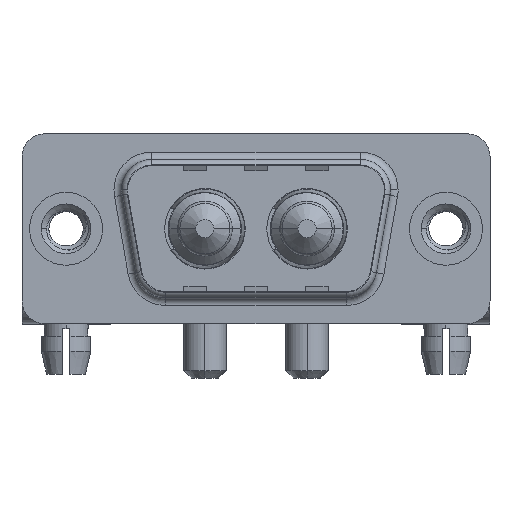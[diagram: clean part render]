
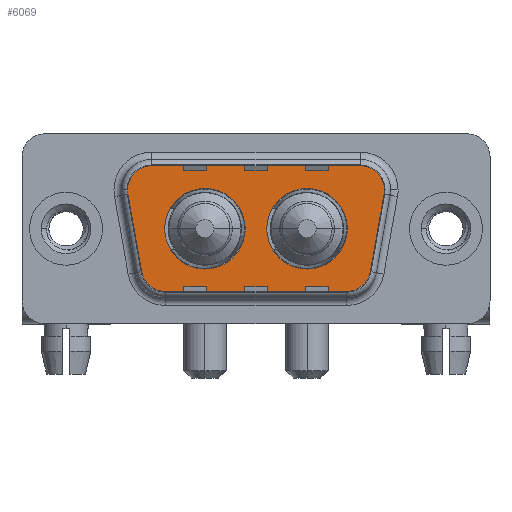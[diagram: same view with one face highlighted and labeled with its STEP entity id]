
A CAD part, top view. The second image highlights one B-rep face of the part: STEP entity #6069.
In plain terms, the highlighted planar face has unit normal (0, 0, 1).
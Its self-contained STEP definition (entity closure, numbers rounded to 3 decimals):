
#270 = CIRCLE ( 'NONE', #10573, 2.65 ) ;
#485 = EDGE_CURVE ( 'NONE', #7321, #1533, #10133, .T. ) ;
#547 = CARTESIAN_POINT ( 'NONE',  ( 9.14, 0., 0. ) ) ;
#634 = VERTEX_POINT ( 'NONE', #9031 ) ;
#652 = AXIS2_PLACEMENT_3D ( 'NONE', #2389, #12251, #5765 ) ;
#685 = CIRCLE ( 'NONE', #13938, 2.65 ) ;
#824 = LINE ( 'NONE', #10684, #3923 ) ;
#887 = DIRECTION ( 'NONE',  ( 0.174, 0.985, 0. ) ) ;
#907 = DIRECTION ( 'NONE',  ( 1., 0., 0. ) ) ;
#1117 = ORIENTED_EDGE ( 'NONE', *, *, #485, .T. ) ;
#1237 = EDGE_CURVE ( 'NONE', #4192, #14026, #5789, .T. ) ;
#1302 = ORIENTED_EDGE ( 'NONE', *, *, #2792, .T. ) ;
#1533 = VERTEX_POINT ( 'NONE', #12613 ) ;
#1662 = ORIENTED_EDGE ( 'NONE', *, *, #10851, .T. ) ;
#1864 = CARTESIAN_POINT ( 'NONE',  ( 18.51, 0., 0. ) ) ;
#2074 = CARTESIAN_POINT ( 'NONE',  ( 9.14, 0., 0. ) ) ;
#2175 = DIRECTION ( 'NONE',  ( -1., 0., 0. ) ) ;
#2204 = DIRECTION ( 'NONE',  ( -1., 0., 0. ) ) ;
#2281 = AXIS2_PLACEMENT_3D ( 'NONE', #3483, #10144, #3620 ) ;
#2372 = DIRECTION ( 'NONE',  ( 0., 0., 1. ) ) ;
#2389 = CARTESIAN_POINT ( 'NONE',  ( 18.541, -2.9, 0. ) ) ;
#2602 = DIRECTION ( 'NONE',  ( 0., 0., 1. ) ) ;
#2766 = CIRCLE ( 'NONE', #13952, 2. ) ;
#2767 = DIRECTION ( 'NONE',  ( 0., 0., 1. ) ) ;
#2792 = EDGE_CURVE ( 'NONE', #11242, #5086, #8557, .T. ) ;
#3089 = EDGE_CURVE ( 'NONE', #634, #4227, #270, .T. ) ;
#3205 = EDGE_LOOP ( 'NONE', ( #7074, #8288 ) ) ;
#3242 = CARTESIAN_POINT ( 'NONE',  ( 19.564, 2.9, 0. ) ) ;
#3483 = CARTESIAN_POINT ( 'NONE',  ( 6.459, -2.9, 0. ) ) ;
#3620 = DIRECTION ( 'NONE',  ( -1., 0., 0. ) ) ;
#3659 = EDGE_CURVE ( 'NONE', #4227, #634, #685, .T. ) ;
#3923 = VECTOR ( 'NONE', #887, 1000. ) ;
#3963 = DIRECTION ( 'NONE',  ( 1., 0., 0. ) ) ;
#4192 = VERTEX_POINT ( 'NONE', #13321 ) ;
#4227 = VERTEX_POINT ( 'NONE', #7830 ) ;
#4237 = EDGE_CURVE ( 'NONE', #5086, #11432, #10915, .T. ) ;
#4302 = CARTESIAN_POINT ( 'NONE',  ( 3.466, 2.553, 0. ) ) ;
#4354 = CIRCLE ( 'NONE', #10530, 2.65 ) ;
#4402 = VERTEX_POINT ( 'NONE', #4816 ) ;
#4488 = LINE ( 'NONE', #11137, #9179 ) ;
#4498 = CARTESIAN_POINT ( 'NONE',  ( 18.541, -4.9, 0. ) ) ;
#4816 = CARTESIAN_POINT ( 'NONE',  ( 21.534, 2.553, 0. ) ) ;
#5084 = AXIS2_PLACEMENT_3D ( 'NONE', #7219, #2767, #7148 ) ;
#5086 = VERTEX_POINT ( 'NONE', #4498 ) ;
#5178 = EDGE_LOOP ( 'NONE', ( #13617, #1662, #7521, #1117, #10846, #5737, #11126, #7976, #1302 ) ) ;
#5289 = VERTEX_POINT ( 'NONE', #11369 ) ;
#5326 = CARTESIAN_POINT ( 'NONE',  ( 19.564, 2.9, 0. ) ) ;
#5380 = VECTOR ( 'NONE', #13698, 1000. ) ;
#5528 = CARTESIAN_POINT ( 'NONE',  ( 21.564, 2.9, 0. ) ) ;
#5575 = DIRECTION ( 'NONE',  ( 0., 0., 1. ) ) ;
#5737 = ORIENTED_EDGE ( 'NONE', *, *, #8093, .T. ) ;
#5765 = DIRECTION ( 'NONE',  ( 1., 0., 0. ) ) ;
#5789 = CIRCLE ( 'NONE', #5084, 2.65 ) ;
#5834 = EDGE_CURVE ( 'NONE', #10342, #6373, #8751, .T. ) ;
#6069 = ADVANCED_FACE ( 'NONE', ( #13302, #6890, #8029 ), #7884, .T. ) ;
#6239 = ORIENTED_EDGE ( 'NONE', *, *, #3089, .F. ) ;
#6373 = VERTEX_POINT ( 'NONE', #11871 ) ;
#6454 = DIRECTION ( 'NONE',  ( 1., 0., 0. ) ) ;
#6860 = CIRCLE ( 'NONE', #2281, 2. ) ;
#6890 = FACE_BOUND ( 'NONE', #7008, .T. ) ;
#7008 = EDGE_LOOP ( 'NONE', ( #6239, #11251 ) ) ;
#7074 = ORIENTED_EDGE ( 'NONE', *, *, #8424, .F. ) ;
#7089 = AXIS2_PLACEMENT_3D ( 'NONE', #10099, #2372, #11249 ) ;
#7148 = DIRECTION ( 'NONE',  ( 1., 0., 0. ) ) ;
#7219 = CARTESIAN_POINT ( 'NONE',  ( 15.86, 0., 0. ) ) ;
#7309 = VECTOR ( 'NONE', #8543, 1000. ) ;
#7321 = VERTEX_POINT ( 'NONE', #5528 ) ;
#7521 = ORIENTED_EDGE ( 'NONE', *, *, #8598, .T. ) ;
#7562 = DIRECTION ( 'NONE',  ( 0., 0., 1. ) ) ;
#7632 = CARTESIAN_POINT ( 'NONE',  ( 5.436, 2.9, 0. ) ) ;
#7729 = EDGE_CURVE ( 'NONE', #6373, #11242, #6860, .T. ) ;
#7830 = CARTESIAN_POINT ( 'NONE',  ( 6.49, 0., 0. ) ) ;
#7884 = PLANE ( 'NONE',  #7089 ) ;
#7976 = ORIENTED_EDGE ( 'NONE', *, *, #7729, .T. ) ;
#8029 = FACE_OUTER_BOUND ( 'NONE', #5178, .T. ) ;
#8093 = EDGE_CURVE ( 'NONE', #5289, #10342, #10751, .T. ) ;
#8122 = DIRECTION ( 'NONE',  ( 1., 0., 0. ) ) ;
#8288 = ORIENTED_EDGE ( 'NONE', *, *, #1237, .F. ) ;
#8424 = EDGE_CURVE ( 'NONE', #14026, #4192, #4354, .T. ) ;
#8473 = CARTESIAN_POINT ( 'NONE',  ( 15.86, 0., 0. ) ) ;
#8481 = CARTESIAN_POINT ( 'NONE',  ( 6.459, -4.9, 0. ) ) ;
#8528 = AXIS2_PLACEMENT_3D ( 'NONE', #5326, #14114, #2175 ) ;
#8543 = DIRECTION ( 'NONE',  ( 0.174, -0.985, 0. ) ) ;
#8557 = LINE ( 'NONE', #8481, #5380 ) ;
#8598 = EDGE_CURVE ( 'NONE', #4402, #7321, #2766, .T. ) ;
#8751 = LINE ( 'NONE', #4302, #7309 ) ;
#9031 = CARTESIAN_POINT ( 'NONE',  ( 11.79, 0., 0. ) ) ;
#9101 = CARTESIAN_POINT ( 'NONE',  ( 20.511, -3.247, 0. ) ) ;
#9179 = VECTOR ( 'NONE', #2204, 1000. ) ;
#9631 = CARTESIAN_POINT ( 'NONE',  ( 3.466, 2.553, 0. ) ) ;
#9898 = DIRECTION ( 'NONE',  ( 0., 0., 1. ) ) ;
#10082 = EDGE_CURVE ( 'NONE', #1533, #5289, #4488, .T. ) ;
#10099 = CARTESIAN_POINT ( 'NONE',  ( 18.541, -2.9, 0. ) ) ;
#10133 = CIRCLE ( 'NONE', #8528, 2. ) ;
#10144 = DIRECTION ( 'NONE',  ( 0., 0., 1. ) ) ;
#10342 = VERTEX_POINT ( 'NONE', #9631 ) ;
#10530 = AXIS2_PLACEMENT_3D ( 'NONE', #8473, #13835, #3963 ) ;
#10573 = AXIS2_PLACEMENT_3D ( 'NONE', #547, #2602, #8122 ) ;
#10684 = CARTESIAN_POINT ( 'NONE',  ( 21.534, 2.553, 0. ) ) ;
#10751 = CIRCLE ( 'NONE', #11653, 2. ) ;
#10846 = ORIENTED_EDGE ( 'NONE', *, *, #10082, .T. ) ;
#10851 = EDGE_CURVE ( 'NONE', #11432, #4402, #824, .T. ) ;
#10915 = CIRCLE ( 'NONE', #652, 2. ) ;
#11126 = ORIENTED_EDGE ( 'NONE', *, *, #5834, .T. ) ;
#11137 = CARTESIAN_POINT ( 'NONE',  ( 5.436, 4.9, 0. ) ) ;
#11242 = VERTEX_POINT ( 'NONE', #11616 ) ;
#11249 = DIRECTION ( 'NONE',  ( 1., 0., 0. ) ) ;
#11251 = ORIENTED_EDGE ( 'NONE', *, *, #3659, .F. ) ;
#11369 = CARTESIAN_POINT ( 'NONE',  ( 5.436, 4.9, 0. ) ) ;
#11432 = VERTEX_POINT ( 'NONE', #9101 ) ;
#11616 = CARTESIAN_POINT ( 'NONE',  ( 6.459, -4.9, 0. ) ) ;
#11653 = AXIS2_PLACEMENT_3D ( 'NONE', #7632, #7562, #907 ) ;
#11871 = CARTESIAN_POINT ( 'NONE',  ( 4.489, -3.247, 0. ) ) ;
#12251 = DIRECTION ( 'NONE',  ( 0., 0., 1. ) ) ;
#12613 = CARTESIAN_POINT ( 'NONE',  ( 19.564, 4.9, 0. ) ) ;
#13302 = FACE_BOUND ( 'NONE', #3205, .T. ) ;
#13321 = CARTESIAN_POINT ( 'NONE',  ( 13.21, 0., 0. ) ) ;
#13617 = ORIENTED_EDGE ( 'NONE', *, *, #4237, .T. ) ;
#13698 = DIRECTION ( 'NONE',  ( 1., 0., 0. ) ) ;
#13835 = DIRECTION ( 'NONE',  ( 0., 0., 1. ) ) ;
#13938 = AXIS2_PLACEMENT_3D ( 'NONE', #2074, #5575, #6454 ) ;
#13952 = AXIS2_PLACEMENT_3D ( 'NONE', #3242, #9898, #14117 ) ;
#14026 = VERTEX_POINT ( 'NONE', #1864 ) ;
#14114 = DIRECTION ( 'NONE',  ( 0., 0., 1. ) ) ;
#14117 = DIRECTION ( 'NONE',  ( -1., 0., 0. ) ) ;
